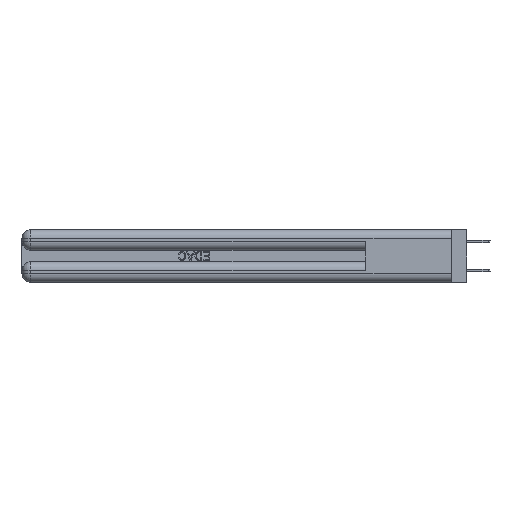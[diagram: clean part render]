
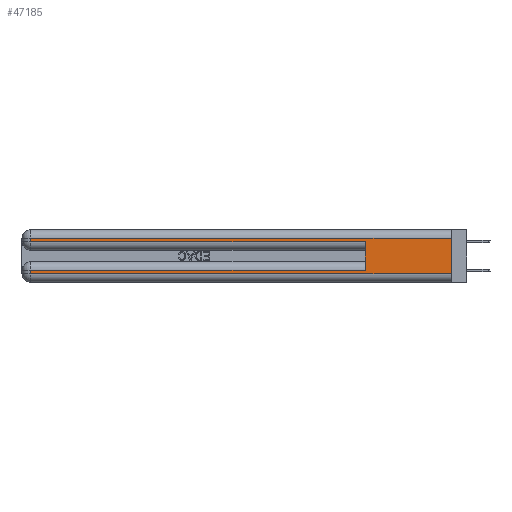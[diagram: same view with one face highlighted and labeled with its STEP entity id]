
A CAD part, left-side view. The second image highlights one B-rep face of the part: STEP entity #47185.
In plain terms, the highlighted planar face has unit normal (-1, 0, 0).
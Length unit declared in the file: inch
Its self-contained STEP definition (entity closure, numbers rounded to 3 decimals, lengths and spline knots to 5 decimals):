
#178 = VERTEX_POINT ( 'NONE', #17547 ) ;
#621 = EDGE_CURVE ( 'NONE', #37922, #47374, #37088, .T. ) ;
#1136 = CARTESIAN_POINT ( 'NONE',  ( 0., 0., 0.285 ) ) ;
#1718 = LINE ( 'NONE', #43890, #37563 ) ;
#2920 = CARTESIAN_POINT ( 'NONE',  ( 0., 0., 0.06 ) ) ;
#3387 = EDGE_CURVE ( 'NONE', #178, #29059, #1718, .T. ) ;
#3495 = CARTESIAN_POINT ( 'NONE',  ( 0., 2.94, 0.37 ) ) ;
#5372 = CARTESIAN_POINT ( 'NONE',  ( 0., 0.6, 0.085 ) ) ;
#5892 = FACE_OUTER_BOUND ( 'NONE', #44121, .T. ) ;
#7718 = DIRECTION ( 'NONE',  ( 0., 0., -1. ) ) ;
#7856 = VECTOR ( 'NONE', #34064, 39.37008 ) ;
#8226 = CARTESIAN_POINT ( 'NONE',  ( 0., 2.94, 0.06 ) ) ;
#9833 = ORIENTED_EDGE ( 'NONE', *, *, #27539, .T. ) ;
#9879 = ORIENTED_EDGE ( 'NONE', *, *, #16965, .F. ) ;
#10457 = CARTESIAN_POINT ( 'NONE',  ( 0., 0., 0.06 ) ) ;
#10905 = LINE ( 'NONE', #20414, #35953 ) ;
#10911 = VECTOR ( 'NONE', #43229, 39.37008 ) ;
#11521 = LINE ( 'NONE', #31459, #49028 ) ;
#11894 = LINE ( 'NONE', #10457, #48782 ) ;
#12640 = ORIENTED_EDGE ( 'NONE', *, *, #3387, .T. ) ;
#12680 = CARTESIAN_POINT ( 'NONE',  ( 0., 2.94, 0.085 ) ) ;
#12735 = DIRECTION ( 'NONE',  ( 0., 0., 1. ) ) ;
#13404 = AXIS2_PLACEMENT_3D ( 'NONE', #42258, #34268, #7718 ) ;
#13809 = VERTEX_POINT ( 'NONE', #5372 ) ;
#13952 = DIRECTION ( 'NONE',  ( 0., -1., 0. ) ) ;
#15003 = LINE ( 'NONE', #44768, #35279 ) ;
#16965 = EDGE_CURVE ( 'NONE', #178, #23207, #10905, .T. ) ;
#17547 = CARTESIAN_POINT ( 'NONE',  ( 0., 0., 0.31 ) ) ;
#18208 = ORIENTED_EDGE ( 'NONE', *, *, #621, .T. ) ;
#19651 = CARTESIAN_POINT ( 'NONE',  ( 0., 0.6, 0.285 ) ) ;
#20414 = CARTESIAN_POINT ( 'NONE',  ( 0., 0., 0.37 ) ) ;
#21646 = VERTEX_POINT ( 'NONE', #46088 ) ;
#23207 = VERTEX_POINT ( 'NONE', #2920 ) ;
#24631 = ORIENTED_EDGE ( 'NONE', *, *, #37192, .F. ) ;
#25679 = DIRECTION ( 'NONE',  ( 0., 0., -1. ) ) ;
#25922 = DIRECTION ( 'NONE',  ( 0., 1., 0. ) ) ;
#27539 = EDGE_CURVE ( 'NONE', #21646, #33956, #42517, .T. ) ;
#28896 = DIRECTION ( 'NONE',  ( 0., 0., -1. ) ) ;
#28904 = EDGE_CURVE ( 'NONE', #47374, #23207, #11894, .T. ) ;
#29059 = VERTEX_POINT ( 'NONE', #45218 ) ;
#30790 = EDGE_CURVE ( 'NONE', #13809, #37922, #34389, .T. ) ;
#30794 = PLANE ( 'NONE',  #13404 ) ;
#31459 = CARTESIAN_POINT ( 'NONE',  ( 0., 0.6, 0.145 ) ) ;
#31688 = ORIENTED_EDGE ( 'NONE', *, *, #28904, .T. ) ;
#33416 = CARTESIAN_POINT ( 'NONE',  ( 0., 0., 0.085 ) ) ;
#33956 = VERTEX_POINT ( 'NONE', #19651 ) ;
#34064 = DIRECTION ( 'NONE',  ( 0., 0., -1. ) ) ;
#34268 = DIRECTION ( 'NONE',  ( 1., 0., 0. ) ) ;
#34389 = LINE ( 'NONE', #33416, #40937 ) ;
#35279 = VECTOR ( 'NONE', #25679, 39.37008 ) ;
#35953 = VECTOR ( 'NONE', #28896, 39.37008 ) ;
#37088 = LINE ( 'NONE', #3495, #7856 ) ;
#37192 = EDGE_CURVE ( 'NONE', #13809, #33956, #11521, .T. ) ;
#37563 = VECTOR ( 'NONE', #44531, 39.37008 ) ;
#37922 = VERTEX_POINT ( 'NONE', #12680 ) ;
#38394 = ORIENTED_EDGE ( 'NONE', *, *, #30790, .T. ) ;
#40937 = VECTOR ( 'NONE', #25922, 39.37008 ) ;
#42236 = ORIENTED_EDGE ( 'NONE', *, *, #45823, .T. ) ;
#42258 = CARTESIAN_POINT ( 'NONE',  ( 0., 0., 0.37 ) ) ;
#42517 = LINE ( 'NONE', #1136, #10911 ) ;
#43229 = DIRECTION ( 'NONE',  ( 0., -1., 0. ) ) ;
#43890 = CARTESIAN_POINT ( 'NONE',  ( 0., 0., 0.31 ) ) ;
#44121 = EDGE_LOOP ( 'NONE', ( #9879, #12640, #42236, #9833, #24631, #38394, #18208, #31688 ) ) ;
#44531 = DIRECTION ( 'NONE',  ( 0., 1., 0. ) ) ;
#44768 = CARTESIAN_POINT ( 'NONE',  ( 0., 2.94, 0.37 ) ) ;
#45218 = CARTESIAN_POINT ( 'NONE',  ( 0., 2.94, 0.31 ) ) ;
#45823 = EDGE_CURVE ( 'NONE', #29059, #21646, #15003, .T. ) ;
#46088 = CARTESIAN_POINT ( 'NONE',  ( 0., 2.94, 0.285 ) ) ;
#47185 = ADVANCED_FACE ( 'NONE', ( #5892 ), #30794, .F. ) ;
#47374 = VERTEX_POINT ( 'NONE', #8226 ) ;
#48782 = VECTOR ( 'NONE', #13952, 39.37008 ) ;
#49028 = VECTOR ( 'NONE', #12735, 39.37008 ) ;
